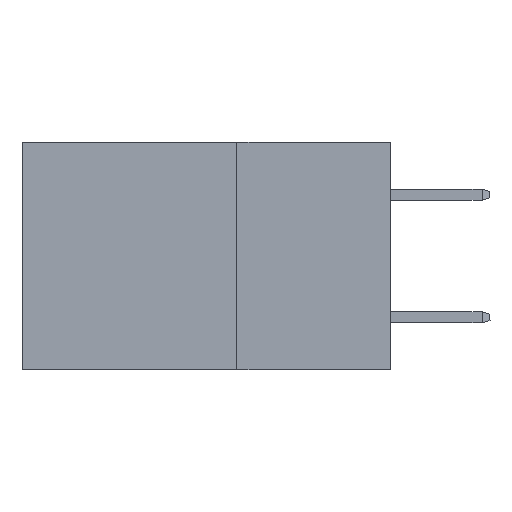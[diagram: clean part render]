
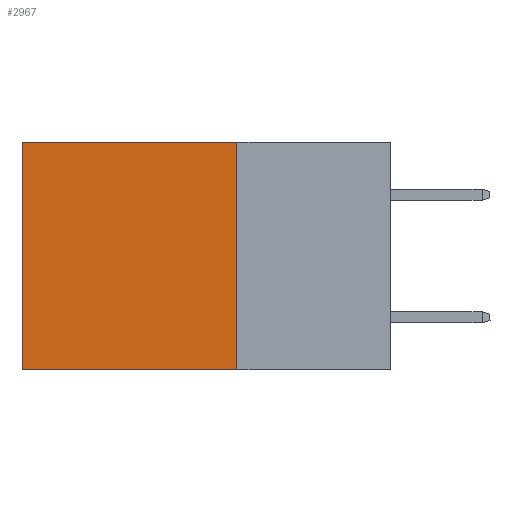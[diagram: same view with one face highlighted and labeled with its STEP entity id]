
A CAD part, left-side view. The second image highlights one B-rep face of the part: STEP entity #2967.
In plain terms, the highlighted planar face has unit normal (-1, 0, 0).
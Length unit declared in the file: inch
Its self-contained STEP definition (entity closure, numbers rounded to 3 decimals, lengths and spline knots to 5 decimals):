
#43 = ORIENTED_EDGE ( 'NONE', *, *, #6784, .T. ) ;
#280 = VECTOR ( 'NONE', #1260, 39.37008 ) ;
#566 = ORIENTED_EDGE ( 'NONE', *, *, #8024, .F. ) ;
#864 = CARTESIAN_POINT ( 'NONE',  ( 0.2875, 0.25, -0.37 ) ) ;
#1032 = CARTESIAN_POINT ( 'NONE',  ( 0.2875, 0.25, -0.37 ) ) ;
#1260 = DIRECTION ( 'NONE',  ( 0., 0., -1. ) ) ;
#1431 = VECTOR ( 'NONE', #2458, 39.37008 ) ;
#1558 = DIRECTION ( 'NONE',  ( 0., 1., 0. ) ) ;
#2065 = CARTESIAN_POINT ( 'NONE',  ( 0.2875, 0.25, 0. ) ) ;
#2188 = EDGE_CURVE ( 'NONE', #3046, #7885, #2916, .T. ) ;
#2204 = LINE ( 'NONE', #864, #7880 ) ;
#2268 = ORIENTED_EDGE ( 'NONE', *, *, #2188, .F. ) ;
#2290 = CARTESIAN_POINT ( 'NONE',  ( 0.2875, 0.25, 0. ) ) ;
#2311 = LINE ( 'NONE', #3947, #6913 ) ;
#2458 = DIRECTION ( 'NONE',  ( 0., 1., 0. ) ) ;
#2865 = PLANE ( 'NONE',  #4110 ) ;
#2916 = LINE ( 'NONE', #4402, #280 ) ;
#2967 = ADVANCED_FACE ( 'NONE', ( #3546 ), #2865, .F. ) ;
#3046 = VERTEX_POINT ( 'NONE', #2065 ) ;
#3546 = FACE_OUTER_BOUND ( 'NONE', #4237, .T. ) ;
#3662 = CARTESIAN_POINT ( 'NONE',  ( 0.2875, 0.25, 0. ) ) ;
#3904 = CARTESIAN_POINT ( 'NONE',  ( 0.2875, 0.6, 0. ) ) ;
#3947 = CARTESIAN_POINT ( 'NONE',  ( 0.2875, 0.6, 0. ) ) ;
#4064 = CARTESIAN_POINT ( 'NONE',  ( 0.2875, 0.6, -0.37 ) ) ;
#4110 = AXIS2_PLACEMENT_3D ( 'NONE', #3662, #7639, #6063 ) ;
#4237 = EDGE_LOOP ( 'NONE', ( #4399, #566, #2268, #43 ) ) ;
#4399 = ORIENTED_EDGE ( 'NONE', *, *, #6812, .T. ) ;
#4402 = CARTESIAN_POINT ( 'NONE',  ( 0.2875, 0.25, 0. ) ) ;
#6063 = DIRECTION ( 'NONE',  ( 0., 0., -1. ) ) ;
#6784 = EDGE_CURVE ( 'NONE', #3046, #8410, #9888, .T. ) ;
#6812 = EDGE_CURVE ( 'NONE', #8410, #7112, #2311, .T. ) ;
#6913 = VECTOR ( 'NONE', #10171, 39.37008 ) ;
#7112 = VERTEX_POINT ( 'NONE', #4064 ) ;
#7639 = DIRECTION ( 'NONE',  ( 1., 0., 0. ) ) ;
#7880 = VECTOR ( 'NONE', #1558, 39.37008 ) ;
#7885 = VERTEX_POINT ( 'NONE', #1032 ) ;
#8024 = EDGE_CURVE ( 'NONE', #7885, #7112, #2204, .T. ) ;
#8410 = VERTEX_POINT ( 'NONE', #3904 ) ;
#9888 = LINE ( 'NONE', #2290, #1431 ) ;
#10171 = DIRECTION ( 'NONE',  ( 0., 0., -1. ) ) ;
